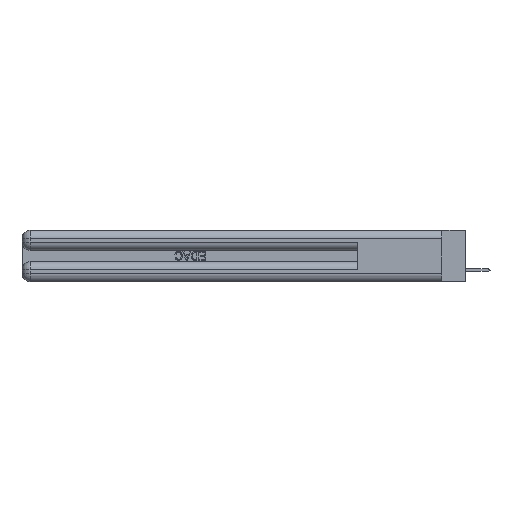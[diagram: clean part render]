
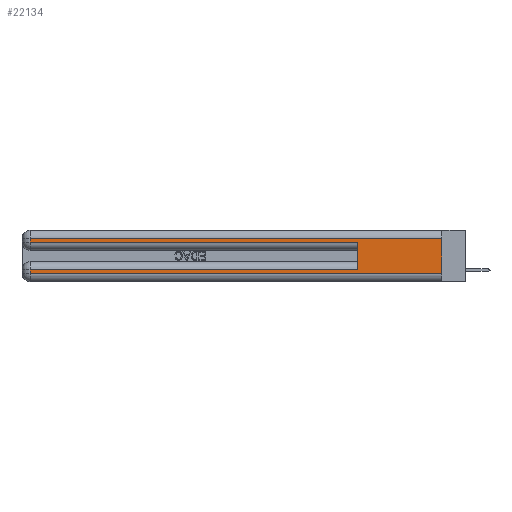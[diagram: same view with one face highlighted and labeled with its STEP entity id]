
A CAD part, left-side view. The second image highlights one B-rep face of the part: STEP entity #22134.
In plain terms, the highlighted planar face has unit normal (-1, 0, 0).
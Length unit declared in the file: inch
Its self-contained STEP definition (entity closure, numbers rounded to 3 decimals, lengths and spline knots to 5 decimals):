
#299 = AXIS2_PLACEMENT_3D ( 'NONE', #19937, #16203, #30824 ) ;
#653 = DIRECTION ( 'NONE',  ( 0., -1., 0. ) ) ;
#2201 = DIRECTION ( 'NONE',  ( 0., 1., 0. ) ) ;
#2544 = CARTESIAN_POINT ( 'NONE',  ( 0., 0., 0.285 ) ) ;
#2834 = CARTESIAN_POINT ( 'NONE',  ( 0., 2.94, 0.37 ) ) ;
#3362 = CARTESIAN_POINT ( 'NONE',  ( 0., 0., 0.06 ) ) ;
#3873 = LINE ( 'NONE', #38524, #35110 ) ;
#4649 = LINE ( 'NONE', #26454, #39272 ) ;
#4867 = EDGE_LOOP ( 'NONE', ( #29210, #31230, #7161, #4907, #45260, #44101, #30130, #5072 ) ) ;
#4907 = ORIENTED_EDGE ( 'NONE', *, *, #23147, .T. ) ;
#5072 = ORIENTED_EDGE ( 'NONE', *, *, #15120, .T. ) ;
#5886 = CARTESIAN_POINT ( 'NONE',  ( 0., 0., 0.085 ) ) ;
#7143 = VECTOR ( 'NONE', #653, 39.37008 ) ;
#7161 = ORIENTED_EDGE ( 'NONE', *, *, #29031, .T. ) ;
#7394 = LINE ( 'NONE', #2544, #35748 ) ;
#13396 = CARTESIAN_POINT ( 'NONE',  ( 0., 2.94, 0.37 ) ) ;
#13696 = VERTEX_POINT ( 'NONE', #29954 ) ;
#14239 = VERTEX_POINT ( 'NONE', #24621 ) ;
#14582 = EDGE_CURVE ( 'NONE', #36231, #35829, #3873, .T. ) ;
#15120 = EDGE_CURVE ( 'NONE', #13696, #44667, #21647, .T. ) ;
#15331 = VECTOR ( 'NONE', #23528, 39.37008 ) ;
#15584 = LINE ( 'NONE', #5886, #45771 ) ;
#16203 = DIRECTION ( 'NONE',  ( 1., 0., 0. ) ) ;
#17809 = EDGE_CURVE ( 'NONE', #40778, #33474, #4649, .T. ) ;
#18059 = CARTESIAN_POINT ( 'NONE',  ( 0., 0., 0.06 ) ) ;
#19220 = LINE ( 'NONE', #13396, #15331 ) ;
#19937 = CARTESIAN_POINT ( 'NONE',  ( 0., 0., 0.37 ) ) ;
#20887 = CARTESIAN_POINT ( 'NONE',  ( 0., 0., 0.37 ) ) ;
#21647 = LINE ( 'NONE', #3362, #7143 ) ;
#21998 = CARTESIAN_POINT ( 'NONE',  ( 0., 0.6, 0.085 ) ) ;
#22134 = ADVANCED_FACE ( 'NONE', ( #32057 ), #30668, .F. ) ;
#23147 = EDGE_CURVE ( 'NONE', #34853, #33474, #7394, .T. ) ;
#23177 = CARTESIAN_POINT ( 'NONE',  ( 0., 0., 0.31 ) ) ;
#23528 = DIRECTION ( 'NONE',  ( 0., 0., -1. ) ) ;
#23856 = DIRECTION ( 'NONE',  ( 0., 1., 0. ) ) ;
#24621 = CARTESIAN_POINT ( 'NONE',  ( 0., 2.94, 0.085 ) ) ;
#26454 = CARTESIAN_POINT ( 'NONE',  ( 0., 0.6, 0.145 ) ) ;
#27641 = DIRECTION ( 'NONE',  ( 0., -1., 0. ) ) ;
#28236 = CARTESIAN_POINT ( 'NONE',  ( 0., 0.6, 0.285 ) ) ;
#28556 = EDGE_CURVE ( 'NONE', #14239, #13696, #39942, .T. ) ;
#29031 = EDGE_CURVE ( 'NONE', #35829, #34853, #19220, .T. ) ;
#29210 = ORIENTED_EDGE ( 'NONE', *, *, #41143, .F. ) ;
#29954 = CARTESIAN_POINT ( 'NONE',  ( 0., 2.94, 0.06 ) ) ;
#30042 = DIRECTION ( 'NONE',  ( 0., 0., 1. ) ) ;
#30130 = ORIENTED_EDGE ( 'NONE', *, *, #28556, .T. ) ;
#30668 = PLANE ( 'NONE',  #299 ) ;
#30824 = DIRECTION ( 'NONE',  ( 0., 0., -1. ) ) ;
#31230 = ORIENTED_EDGE ( 'NONE', *, *, #14582, .T. ) ;
#31663 = DIRECTION ( 'NONE',  ( 0., 0., -1. ) ) ;
#32057 = FACE_OUTER_BOUND ( 'NONE', #4867, .T. ) ;
#33474 = VERTEX_POINT ( 'NONE', #28236 ) ;
#34853 = VERTEX_POINT ( 'NONE', #36217 ) ;
#35043 = CARTESIAN_POINT ( 'NONE',  ( 0., 2.94, 0.31 ) ) ;
#35110 = VECTOR ( 'NONE', #2201, 39.37008 ) ;
#35748 = VECTOR ( 'NONE', #27641, 39.37008 ) ;
#35829 = VERTEX_POINT ( 'NONE', #35043 ) ;
#36217 = CARTESIAN_POINT ( 'NONE',  ( 0., 2.94, 0.285 ) ) ;
#36231 = VERTEX_POINT ( 'NONE', #23177 ) ;
#38524 = CARTESIAN_POINT ( 'NONE',  ( 0., 0., 0.31 ) ) ;
#39188 = VECTOR ( 'NONE', #41962, 39.37008 ) ;
#39272 = VECTOR ( 'NONE', #30042, 39.37008 ) ;
#39942 = LINE ( 'NONE', #2834, #43885 ) ;
#40778 = VERTEX_POINT ( 'NONE', #21998 ) ;
#41143 = EDGE_CURVE ( 'NONE', #36231, #44667, #42039, .T. ) ;
#41962 = DIRECTION ( 'NONE',  ( 0., 0., -1. ) ) ;
#42039 = LINE ( 'NONE', #20887, #39188 ) ;
#43824 = EDGE_CURVE ( 'NONE', #40778, #14239, #15584, .T. ) ;
#43885 = VECTOR ( 'NONE', #31663, 39.37008 ) ;
#44101 = ORIENTED_EDGE ( 'NONE', *, *, #43824, .T. ) ;
#44667 = VERTEX_POINT ( 'NONE', #18059 ) ;
#45260 = ORIENTED_EDGE ( 'NONE', *, *, #17809, .F. ) ;
#45771 = VECTOR ( 'NONE', #23856, 39.37008 ) ;
